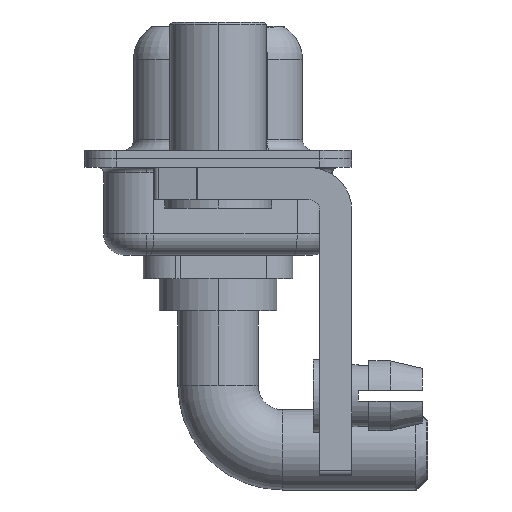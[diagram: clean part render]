
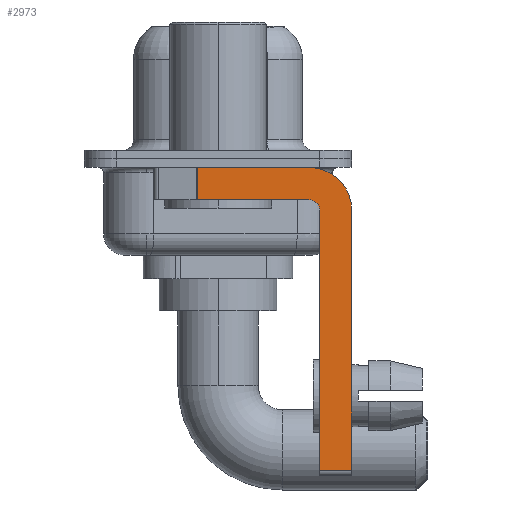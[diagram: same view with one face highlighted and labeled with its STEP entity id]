
A CAD part, left-side view. The second image highlights one B-rep face of the part: STEP entity #2973.
In plain terms, the highlighted planar face has unit normal (-1, 0, 0).
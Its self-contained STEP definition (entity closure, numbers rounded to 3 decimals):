
#145 = LINE ( 'NONE', #12935, #14317 ) ;
#330 = DIRECTION ( 'NONE',  ( 0., -1., 0. ) ) ;
#411 = LINE ( 'NONE', #12575, #5751 ) ;
#470 = EDGE_CURVE ( 'NONE', #6493, #4033, #3796, .T. ) ;
#824 = VERTEX_POINT ( 'NONE', #9532 ) ;
#1292 = DIRECTION ( 'NONE',  ( 0., 0., -1. ) ) ;
#1336 = CARTESIAN_POINT ( 'NONE',  ( -2.9, -4.25, -14.55 ) ) ;
#1393 = CARTESIAN_POINT ( 'NONE',  ( -2.9, -4.25, -2.4 ) ) ;
#1540 = EDGE_CURVE ( 'NONE', #16914, #1722, #145, .T. ) ;
#1722 = VERTEX_POINT ( 'NONE', #13288 ) ;
#2362 = CARTESIAN_POINT ( 'NONE',  ( -2.9, -4.75, -2.4 ) ) ;
#2651 = LINE ( 'NONE', #8211, #14303 ) ;
#2973 = ADVANCED_FACE ( 'NONE', ( #4587 ), #8777, .F. ) ;
#3091 = ORIENTED_EDGE ( 'NONE', *, *, #470, .F. ) ;
#3158 = ORIENTED_EDGE ( 'NONE', *, *, #1540, .F. ) ;
#3466 = DIRECTION ( 'NONE',  ( 0., 0., -1. ) ) ;
#3796 = LINE ( 'NONE', #16073, #17421 ) ;
#3949 = CARTESIAN_POINT ( 'NONE',  ( -2.9, -6.25, -14.55 ) ) ;
#4033 = VERTEX_POINT ( 'NONE', #16429 ) ;
#4519 = LINE ( 'NONE', #1336, #15464 ) ;
#4579 = CARTESIAN_POINT ( 'NONE',  ( -2.9, -6.25, -2.4 ) ) ;
#4587 = FACE_OUTER_BOUND ( 'NONE', #5484, .T. ) ;
#4652 = LINE ( 'NONE', #10110, #5613 ) ;
#5484 = EDGE_LOOP ( 'NONE', ( #3158, #8177, #3091, #11230, #16451, #13701, #17619, #9152 ) ) ;
#5613 = VECTOR ( 'NONE', #3466, 1000. ) ;
#5664 = AXIS2_PLACEMENT_3D ( 'NONE', #6063, #15743, #8875 ) ;
#5751 = VECTOR ( 'NONE', #17001, 1000. ) ;
#5985 = EDGE_CURVE ( 'NONE', #1722, #10704, #16518, .T. ) ;
#6063 = CARTESIAN_POINT ( 'NONE',  ( -2.9, -4.25, -2.4 ) ) ;
#6493 = VERTEX_POINT ( 'NONE', #7053 ) ;
#6781 = DIRECTION ( 'NONE',  ( 0., 0., 1. ) ) ;
#7053 = CARTESIAN_POINT ( 'NONE',  ( -2.9, -4.25, -1.9 ) ) ;
#7786 = VERTEX_POINT ( 'NONE', #2362 ) ;
#7825 = DIRECTION ( 'NONE',  ( 0., 1., 0. ) ) ;
#8177 = ORIENTED_EDGE ( 'NONE', *, *, #10933, .T. ) ;
#8211 = CARTESIAN_POINT ( 'NONE',  ( -2.9, 0.978, -1.9 ) ) ;
#8777 = PLANE ( 'NONE',  #5664 ) ;
#8789 = VERTEX_POINT ( 'NONE', #3949 ) ;
#8827 = EDGE_CURVE ( 'NONE', #7786, #6493, #13950, .T. ) ;
#8875 = DIRECTION ( 'NONE',  ( 0., 0., -1. ) ) ;
#9152 = ORIENTED_EDGE ( 'NONE', *, *, #5985, .F. ) ;
#9532 = CARTESIAN_POINT ( 'NONE',  ( -2.9, -4.75, -14.55 ) ) ;
#10110 = CARTESIAN_POINT ( 'NONE',  ( -2.9, -6.25, -2.4 ) ) ;
#10704 = VERTEX_POINT ( 'NONE', #4579 ) ;
#10933 = EDGE_CURVE ( 'NONE', #16914, #4033, #2651, .T. ) ;
#11230 = ORIENTED_EDGE ( 'NONE', *, *, #8827, .F. ) ;
#11928 = EDGE_CURVE ( 'NONE', #824, #8789, #4519, .T. ) ;
#12405 = DIRECTION ( 'NONE',  ( 1., 0., 0. ) ) ;
#12476 = DIRECTION ( 'NONE',  ( -1., 0., 0. ) ) ;
#12490 = CARTESIAN_POINT ( 'NONE',  ( -2.9, -4.25, -2.4 ) ) ;
#12575 = CARTESIAN_POINT ( 'NONE',  ( -2.9, -4.75, -14.8 ) ) ;
#12661 = DIRECTION ( 'NONE',  ( 0., -1., 0. ) ) ;
#12738 = AXIS2_PLACEMENT_3D ( 'NONE', #12490, #12405, #15291 ) ;
#12935 = CARTESIAN_POINT ( 'NONE',  ( -2.9, 3., -0.4 ) ) ;
#13288 = CARTESIAN_POINT ( 'NONE',  ( -2.9, -4.25, -0.4 ) ) ;
#13701 = ORIENTED_EDGE ( 'NONE', *, *, #11928, .T. ) ;
#13950 = CIRCLE ( 'NONE', #17695, 0.5 ) ;
#14303 = VECTOR ( 'NONE', #1292, 1000. ) ;
#14317 = VECTOR ( 'NONE', #12661, 1000. ) ;
#15291 = DIRECTION ( 'NONE',  ( 0., 0., -1. ) ) ;
#15464 = VECTOR ( 'NONE', #330, 1000. ) ;
#15743 = DIRECTION ( 'NONE',  ( 1., 0., 0. ) ) ;
#16073 = CARTESIAN_POINT ( 'NONE',  ( -2.9, -4.25, -1.9 ) ) ;
#16429 = CARTESIAN_POINT ( 'NONE',  ( -2.9, 0.978, -1.9 ) ) ;
#16451 = ORIENTED_EDGE ( 'NONE', *, *, #16844, .F. ) ;
#16518 = CIRCLE ( 'NONE', #12738, 2. ) ;
#16825 = CARTESIAN_POINT ( 'NONE',  ( -2.9, 0.978, -0.4 ) ) ;
#16844 = EDGE_CURVE ( 'NONE', #824, #7786, #411, .T. ) ;
#16914 = VERTEX_POINT ( 'NONE', #16825 ) ;
#17001 = DIRECTION ( 'NONE',  ( 0., 0., 1. ) ) ;
#17421 = VECTOR ( 'NONE', #7825, 1000. ) ;
#17439 = EDGE_CURVE ( 'NONE', #10704, #8789, #4652, .T. ) ;
#17619 = ORIENTED_EDGE ( 'NONE', *, *, #17439, .F. ) ;
#17695 = AXIS2_PLACEMENT_3D ( 'NONE', #1393, #12476, #6781 ) ;
